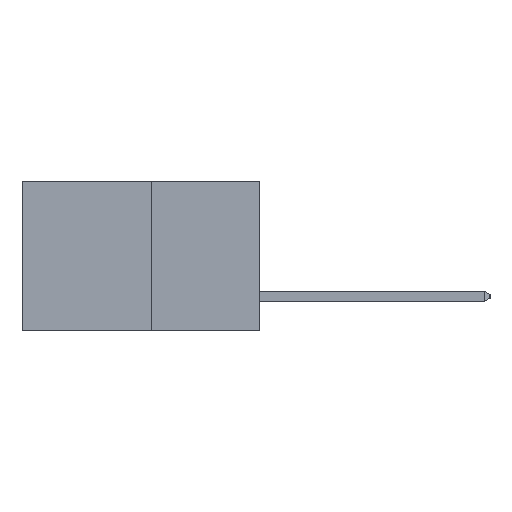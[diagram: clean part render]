
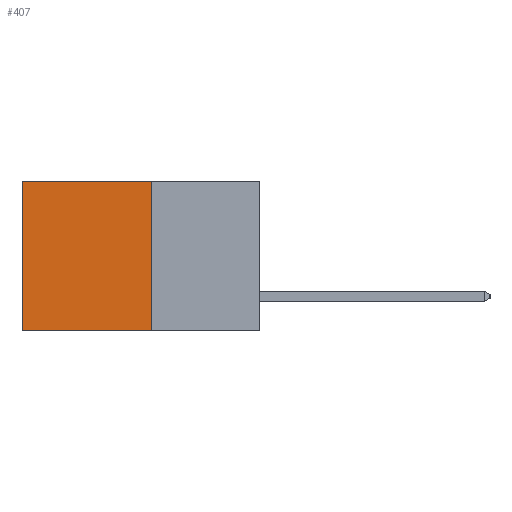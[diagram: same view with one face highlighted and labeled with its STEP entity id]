
A CAD part, left-side view. The second image highlights one B-rep face of the part: STEP entity #407.
In plain terms, the highlighted planar face has unit normal (-1, 0, 0).
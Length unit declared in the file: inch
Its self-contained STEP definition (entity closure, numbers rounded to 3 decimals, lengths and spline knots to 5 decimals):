
#11 = VERTEX_POINT ( 'NONE', #8818 ) ;
#51 = LINE ( 'NONE', #6579, #12174 ) ;
#175 = CARTESIAN_POINT ( 'NONE',  ( 0.277, 0.27, 0. ) ) ;
#407 = ADVANCED_FACE ( 'NONE', ( #4284 ), #13514, .F. ) ;
#873 = VECTOR ( 'NONE', #2954, 39.37008 ) ;
#1271 = LINE ( 'NONE', #1491, #873 ) ;
#1491 = CARTESIAN_POINT ( 'NONE',  ( 0.277, 0.27, -0.37 ) ) ;
#2954 = DIRECTION ( 'NONE',  ( 0., 1., 0. ) ) ;
#3647 = DIRECTION ( 'NONE',  ( 0., 1., 0. ) ) ;
#4284 = FACE_OUTER_BOUND ( 'NONE', #9643, .T. ) ;
#4365 = CARTESIAN_POINT ( 'NONE',  ( 0.277, 0.27, -0.37 ) ) ;
#4523 = VECTOR ( 'NONE', #8916, 39.37008 ) ;
#4577 = EDGE_CURVE ( 'NONE', #6162, #8660, #1271, .T. ) ;
#4948 = LINE ( 'NONE', #9324, #10619 ) ;
#4952 = EDGE_CURVE ( 'NONE', #11, #8660, #12854, .T. ) ;
#5494 = CARTESIAN_POINT ( 'NONE',  ( 0.277, 0.27, -0.37 ) ) ;
#6081 = ORIENTED_EDGE ( 'NONE', *, *, #10001, .F. ) ;
#6162 = VERTEX_POINT ( 'NONE', #4365 ) ;
#6422 = VERTEX_POINT ( 'NONE', #175 ) ;
#6459 = ORIENTED_EDGE ( 'NONE', *, *, #4577, .F. ) ;
#6579 = CARTESIAN_POINT ( 'NONE',  ( 0.277, 0.27, -0.37 ) ) ;
#8630 = CARTESIAN_POINT ( 'NONE',  ( 0.277, 0.59, -0.37 ) ) ;
#8660 = VERTEX_POINT ( 'NONE', #8630 ) ;
#8791 = DIRECTION ( 'NONE',  ( 0., 0., -1. ) ) ;
#8818 = CARTESIAN_POINT ( 'NONE',  ( 0.277, 0.59, 0. ) ) ;
#8916 = DIRECTION ( 'NONE',  ( 0., 0., -1. ) ) ;
#8923 = CARTESIAN_POINT ( 'NONE',  ( 0.277, 0.59, -0.37 ) ) ;
#9324 = CARTESIAN_POINT ( 'NONE',  ( 0.277, 0.27, 0. ) ) ;
#9643 = EDGE_LOOP ( 'NONE', ( #14663, #6459, #6081, #10115 ) ) ;
#10001 = EDGE_CURVE ( 'NONE', #6422, #6162, #51, .T. ) ;
#10115 = ORIENTED_EDGE ( 'NONE', *, *, #12954, .T. ) ;
#10619 = VECTOR ( 'NONE', #3647, 39.37008 ) ;
#11738 = DIRECTION ( 'NONE',  ( 1., 0., 0. ) ) ;
#12146 = AXIS2_PLACEMENT_3D ( 'NONE', #5494, #11738, #14536 ) ;
#12174 = VECTOR ( 'NONE', #8791, 39.37008 ) ;
#12854 = LINE ( 'NONE', #8923, #4523 ) ;
#12954 = EDGE_CURVE ( 'NONE', #6422, #11, #4948, .T. ) ;
#13514 = PLANE ( 'NONE',  #12146 ) ;
#14536 = DIRECTION ( 'NONE',  ( 0., 0., -1. ) ) ;
#14663 = ORIENTED_EDGE ( 'NONE', *, *, #4952, .T. ) ;
